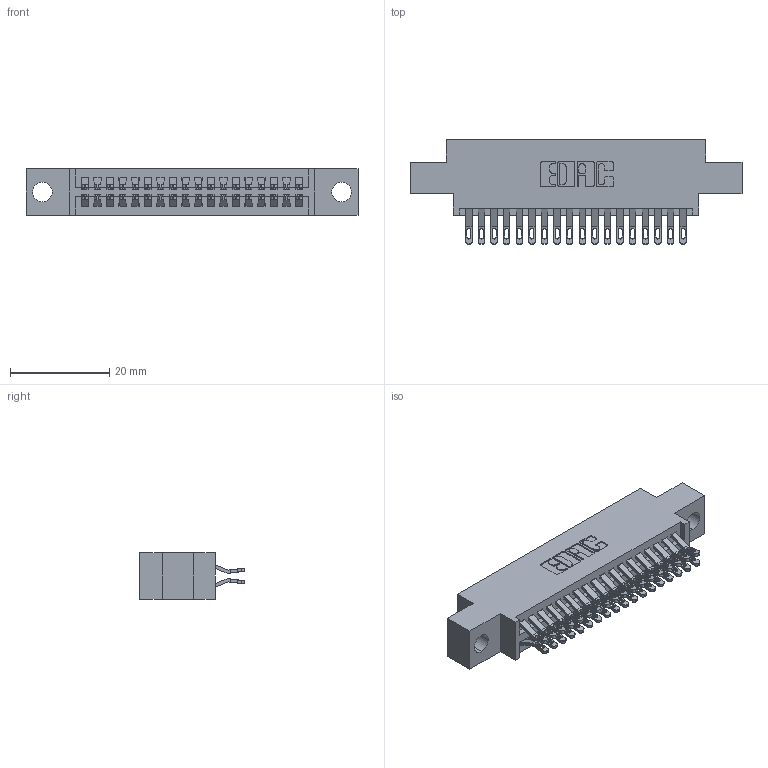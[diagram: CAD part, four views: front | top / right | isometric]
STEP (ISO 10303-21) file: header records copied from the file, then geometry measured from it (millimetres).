
FILE_DESCRIPTION (( 'STEP AP203' ), '1' );
FILE_NAME ('345-036-555-804.STEP', '2021-05-20T00:31:24', ( '' ), ( '' ), 'SwSTEP 2.0', 'SolidWorks 2020', '' );
FILE_SCHEMA (( 'CONFIG_CONTROL_DESIGN' ));
Length unit declared in the file: inch
Products named in the file (3): 345-036-555-804; 345 Part_0.170 Offset - 0.156 Dia-TI; 345-292-001_555 Tail
Assembly tree (37 placements, depth 2):
  345-036-555-804
    345 Part_0.170 Offset - 0.156 Dia-TI
    345-292-001_555 Tail  x36
Bounding box: 66.93 x 21.13 x 9.4 mm (x, y, z)
Volume: 6163.9 mm3; surface area: 9004.6 mm2
Topology: 37 solids, 37 shells, 2160 faces, 6761 edges, 4506 vertices
Faces by surface type: plane 1214, cylinder 946
Entity records: 18231 total; most frequent: CARTESIAN_POINT 3120, ORIENTED_EDGE 3022, DIRECTION 2747, EDGE_CURVE 1511, LINE 1287, VECTOR 1287, VERTEX_POINT 1006, AXIS2_PLACEMENT_3D 730
